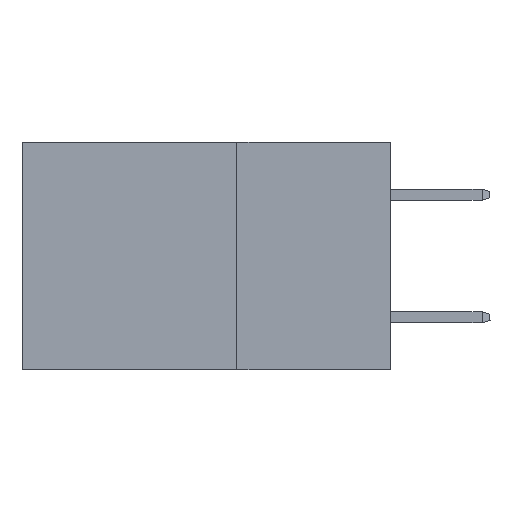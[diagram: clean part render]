
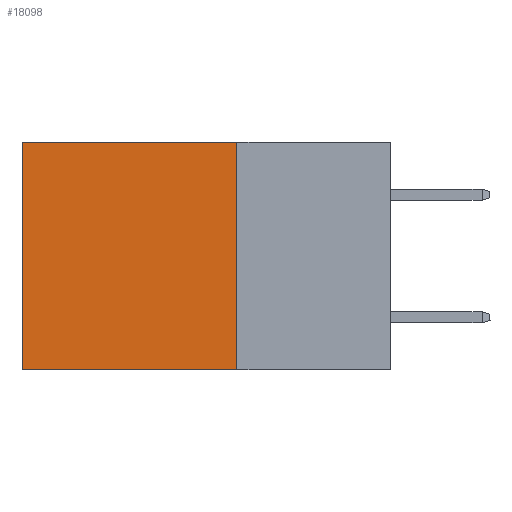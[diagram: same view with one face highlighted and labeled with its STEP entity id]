
A CAD part, left-side view. The second image highlights one B-rep face of the part: STEP entity #18098.
In plain terms, the highlighted planar face has unit normal (-1, 0, 0).
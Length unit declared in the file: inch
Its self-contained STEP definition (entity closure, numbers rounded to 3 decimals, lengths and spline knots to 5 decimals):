
#1063 = LINE ( 'NONE', #3342, #22317 ) ;
#1206 = ORIENTED_EDGE ( 'NONE', *, *, #1880, .F. ) ;
#1880 = EDGE_CURVE ( 'NONE', #13006, #30364, #16558, .T. ) ;
#2186 = CARTESIAN_POINT ( 'NONE',  ( 0.2875, 0.25, -0.37 ) ) ;
#2421 = DIRECTION ( 'NONE',  ( 0., 0., -1. ) ) ;
#3342 = CARTESIAN_POINT ( 'NONE',  ( 0.2875, 0.25, 0. ) ) ;
#3514 = EDGE_CURVE ( 'NONE', #5575, #13006, #1063, .T. ) ;
#5575 = VERTEX_POINT ( 'NONE', #11762 ) ;
#7013 = PLANE ( 'NONE',  #25167 ) ;
#7870 = DIRECTION ( 'NONE',  ( 0., 0., -1. ) ) ;
#8602 = VECTOR ( 'NONE', #28936, 39.37008 ) ;
#9953 = LINE ( 'NONE', #31923, #23037 ) ;
#10371 = VECTOR ( 'NONE', #7870, 39.37008 ) ;
#11639 = CARTESIAN_POINT ( 'NONE',  ( 0.2875, 0.25, -0.37 ) ) ;
#11762 = CARTESIAN_POINT ( 'NONE',  ( 0.2875, 0.25, 0. ) ) ;
#11865 = EDGE_CURVE ( 'NONE', #22244, #30364, #24670, .T. ) ;
#12720 = DIRECTION ( 'NONE',  ( 1., 0., 0. ) ) ;
#13006 = VERTEX_POINT ( 'NONE', #11639 ) ;
#13437 = CARTESIAN_POINT ( 'NONE',  ( 0.2875, 0.6, -0.37 ) ) ;
#15204 = CARTESIAN_POINT ( 'NONE',  ( 0.2875, 0.6, 0. ) ) ;
#16558 = LINE ( 'NONE', #2186, #8602 ) ;
#16631 = ORIENTED_EDGE ( 'NONE', *, *, #11865, .T. ) ;
#17678 = EDGE_CURVE ( 'NONE', #5575, #22244, #9953, .T. ) ;
#18098 = ADVANCED_FACE ( 'NONE', ( #24944 ), #7013, .F. ) ;
#19725 = DIRECTION ( 'NONE',  ( 0., 1., 0. ) ) ;
#19841 = EDGE_LOOP ( 'NONE', ( #16631, #1206, #26931, #25330 ) ) ;
#22244 = VERTEX_POINT ( 'NONE', #30180 ) ;
#22317 = VECTOR ( 'NONE', #28441, 39.37008 ) ;
#23037 = VECTOR ( 'NONE', #19725, 39.37008 ) ;
#24670 = LINE ( 'NONE', #15204, #10371 ) ;
#24944 = FACE_OUTER_BOUND ( 'NONE', #19841, .T. ) ;
#25167 = AXIS2_PLACEMENT_3D ( 'NONE', #29962, #12720, #2421 ) ;
#25330 = ORIENTED_EDGE ( 'NONE', *, *, #17678, .T. ) ;
#26931 = ORIENTED_EDGE ( 'NONE', *, *, #3514, .F. ) ;
#28441 = DIRECTION ( 'NONE',  ( 0., 0., -1. ) ) ;
#28936 = DIRECTION ( 'NONE',  ( 0., 1., 0. ) ) ;
#29962 = CARTESIAN_POINT ( 'NONE',  ( 0.2875, 0.25, 0. ) ) ;
#30180 = CARTESIAN_POINT ( 'NONE',  ( 0.2875, 0.6, 0. ) ) ;
#30364 = VERTEX_POINT ( 'NONE', #13437 ) ;
#31923 = CARTESIAN_POINT ( 'NONE',  ( 0.2875, 0.25, 0. ) ) ;
